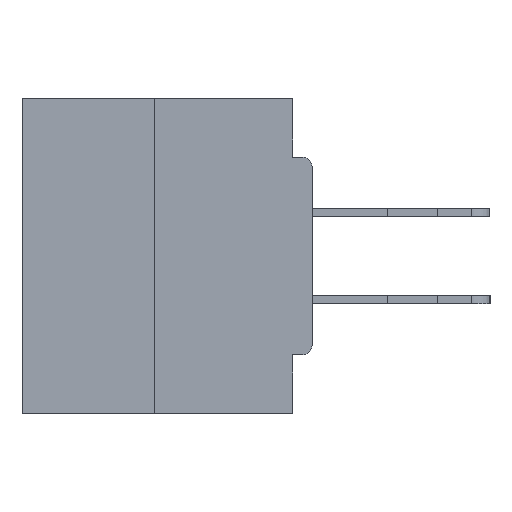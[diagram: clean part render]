
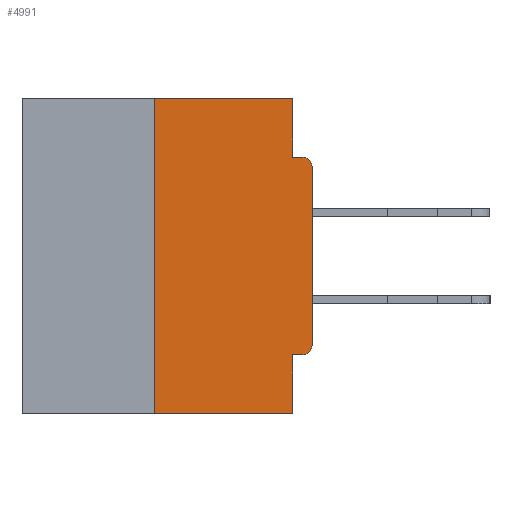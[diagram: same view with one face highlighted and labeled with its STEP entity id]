
A CAD part, left-side view. The second image highlights one B-rep face of the part: STEP entity #4991.
In plain terms, the highlighted planar face has unit normal (-1, 0, 0).
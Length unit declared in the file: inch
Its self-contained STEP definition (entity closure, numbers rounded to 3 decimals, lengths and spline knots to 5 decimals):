
#195 = VERTEX_POINT ( 'NONE', #23004 ) ;
#337 = DIRECTION ( 'NONE',  ( 0., 0., -1. ) ) ;
#418 = DIRECTION ( 'NONE',  ( 0., 0., 1. ) ) ;
#667 = CARTESIAN_POINT ( 'NONE',  ( 0., 0.46, -0.5 ) ) ;
#714 = ORIENTED_EDGE ( 'NONE', *, *, #31205, .T. ) ;
#1572 = VECTOR ( 'NONE', #4733, 39.37008 ) ;
#1667 = ORIENTED_EDGE ( 'NONE', *, *, #10042, .F. ) ;
#2839 = CARTESIAN_POINT ( 'NONE',  ( 0., 0.031, -0.4065 ) ) ;
#3411 = VERTEX_POINT ( 'NONE', #16461 ) ;
#3759 = CARTESIAN_POINT ( 'NONE',  ( 0., 0.25, 0. ) ) ;
#4710 = VERTEX_POINT ( 'NONE', #28439 ) ;
#4733 = DIRECTION ( 'NONE',  ( 0., -1., 0. ) ) ;
#4991 = ADVANCED_FACE ( 'NONE', ( #7160 ), #37496, .F. ) ;
#5162 = AXIS2_PLACEMENT_3D ( 'NONE', #30006, #43610, #12724 ) ;
#5500 = ORIENTED_EDGE ( 'NONE', *, *, #13384, .F. ) ;
#6005 = VECTOR ( 'NONE', #30102, 39.37008 ) ;
#6422 = CARTESIAN_POINT ( 'NONE',  ( 0., 0., -0.4065 ) ) ;
#7157 = CIRCLE ( 'NONE', #5162, 0.015 ) ;
#7160 = FACE_OUTER_BOUND ( 'NONE', #20639, .T. ) ;
#7190 = DIRECTION ( 'NONE',  ( 0., 0., 1. ) ) ;
#8043 = DIRECTION ( 'NONE',  ( -1., 0., 0. ) ) ;
#9290 = CARTESIAN_POINT ( 'NONE',  ( 0., 0.031, 0. ) ) ;
#9828 = VERTEX_POINT ( 'NONE', #38562 ) ;
#10042 = EDGE_CURVE ( 'NONE', #4710, #13277, #42361, .T. ) ;
#10113 = VERTEX_POINT ( 'NONE', #34578 ) ;
#10465 = CARTESIAN_POINT ( 'NONE',  ( 0., 0.031, 0. ) ) ;
#10879 = DIRECTION ( 'NONE',  ( 0., -1., 0. ) ) ;
#10957 = VECTOR ( 'NONE', #40697, 39.37008 ) ;
#12503 = AXIS2_PLACEMENT_3D ( 'NONE', #25341, #8043, #15045 ) ;
#12724 = DIRECTION ( 'NONE',  ( 0., 0., -1. ) ) ;
#13277 = VERTEX_POINT ( 'NONE', #2839 ) ;
#13384 = EDGE_CURVE ( 'NONE', #9828, #36785, #38854, .T. ) ;
#15045 = DIRECTION ( 'NONE',  ( 0., 0., -1. ) ) ;
#16461 = CARTESIAN_POINT ( 'NONE',  ( 0., 0., -0.1085 ) ) ;
#17078 = CARTESIAN_POINT ( 'NONE',  ( 0., 0.031, -0.5 ) ) ;
#18410 = CARTESIAN_POINT ( 'NONE',  ( 0., 0., -0.0935 ) ) ;
#18903 = ORIENTED_EDGE ( 'NONE', *, *, #30468, .F. ) ;
#19222 = VECTOR ( 'NONE', #418, 39.37008 ) ;
#19474 = LINE ( 'NONE', #18410, #1572 ) ;
#20314 = LINE ( 'NONE', #3759, #19222 ) ;
#20496 = VERTEX_POINT ( 'NONE', #22213 ) ;
#20639 = EDGE_LOOP ( 'NONE', ( #5500, #22636, #714, #18903, #1667, #35587, #44071, #40768, #39744, #39595 ) ) ;
#20717 = CARTESIAN_POINT ( 'NONE',  ( 0., 0., 0. ) ) ;
#22213 = CARTESIAN_POINT ( 'NONE',  ( 0., 0.031, -0.5 ) ) ;
#22636 = ORIENTED_EDGE ( 'NONE', *, *, #26265, .F. ) ;
#23004 = CARTESIAN_POINT ( 'NONE',  ( 0., 0., -0.3915 ) ) ;
#23492 = EDGE_CURVE ( 'NONE', #32385, #38682, #19474, .T. ) ;
#23598 = CARTESIAN_POINT ( 'NONE',  ( 0., 0.015, -0.0935 ) ) ;
#23614 = VECTOR ( 'NONE', #337, 39.37008 ) ;
#25341 = CARTESIAN_POINT ( 'NONE',  ( 0., 0.015, -0.3915 ) ) ;
#26265 = EDGE_CURVE ( 'NONE', #10113, #9828, #20314, .T. ) ;
#26885 = CARTESIAN_POINT ( 'NONE',  ( 0., 0.031, -0.0935 ) ) ;
#27049 = VECTOR ( 'NONE', #7190, 39.37008 ) ;
#27321 = EDGE_CURVE ( 'NONE', #3411, #38682, #7157, .T. ) ;
#27459 = EDGE_CURVE ( 'NONE', #36785, #32385, #32108, .T. ) ;
#28439 = CARTESIAN_POINT ( 'NONE',  ( 0., 0.015, -0.4065 ) ) ;
#29071 = CARTESIAN_POINT ( 'NONE',  ( 0., 0.46, 0. ) ) ;
#29694 = EDGE_CURVE ( 'NONE', #4710, #195, #44824, .T. ) ;
#30006 = CARTESIAN_POINT ( 'NONE',  ( 0., 0.015, -0.1085 ) ) ;
#30102 = DIRECTION ( 'NONE',  ( 0., 1., 0. ) ) ;
#30415 = DIRECTION ( 'NONE',  ( 1., 0., 0. ) ) ;
#30468 = EDGE_CURVE ( 'NONE', #13277, #20496, #32841, .T. ) ;
#31205 = EDGE_CURVE ( 'NONE', #10113, #20496, #44651, .T. ) ;
#32108 = LINE ( 'NONE', #9290, #10957 ) ;
#32385 = VERTEX_POINT ( 'NONE', #26885 ) ;
#32841 = LINE ( 'NONE', #17078, #23614 ) ;
#33888 = EDGE_CURVE ( 'NONE', #195, #3411, #44929, .T. ) ;
#34578 = CARTESIAN_POINT ( 'NONE',  ( 0., 0.25, -0.5 ) ) ;
#35587 = ORIENTED_EDGE ( 'NONE', *, *, #29694, .T. ) ;
#35858 = DIRECTION ( 'NONE',  ( 0., -1., 0. ) ) ;
#36785 = VERTEX_POINT ( 'NONE', #10465 ) ;
#37344 = DIRECTION ( 'NONE',  ( 0., 0., -1. ) ) ;
#37496 = PLANE ( 'NONE',  #38868 ) ;
#37802 = CARTESIAN_POINT ( 'NONE',  ( 0., 0.46, 0. ) ) ;
#38303 = VECTOR ( 'NONE', #35858, 39.37008 ) ;
#38562 = CARTESIAN_POINT ( 'NONE',  ( 0., 0.25, 0. ) ) ;
#38682 = VERTEX_POINT ( 'NONE', #23598 ) ;
#38854 = LINE ( 'NONE', #29071, #38303 ) ;
#38868 = AXIS2_PLACEMENT_3D ( 'NONE', #37802, #30415, #37344 ) ;
#39225 = VECTOR ( 'NONE', #10879, 39.37008 ) ;
#39595 = ORIENTED_EDGE ( 'NONE', *, *, #27459, .F. ) ;
#39744 = ORIENTED_EDGE ( 'NONE', *, *, #23492, .F. ) ;
#40697 = DIRECTION ( 'NONE',  ( 0., 0., -1. ) ) ;
#40768 = ORIENTED_EDGE ( 'NONE', *, *, #27321, .T. ) ;
#42361 = LINE ( 'NONE', #6422, #6005 ) ;
#43610 = DIRECTION ( 'NONE',  ( -1., 0., 0. ) ) ;
#44071 = ORIENTED_EDGE ( 'NONE', *, *, #33888, .T. ) ;
#44651 = LINE ( 'NONE', #667, #39225 ) ;
#44824 = CIRCLE ( 'NONE', #12503, 0.015 ) ;
#44929 = LINE ( 'NONE', #20717, #27049 ) ;
